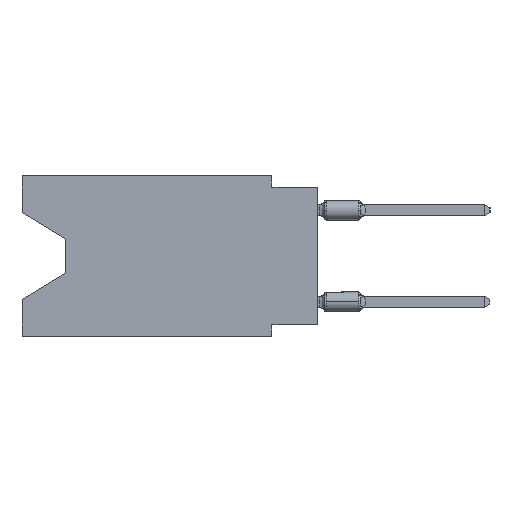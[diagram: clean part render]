
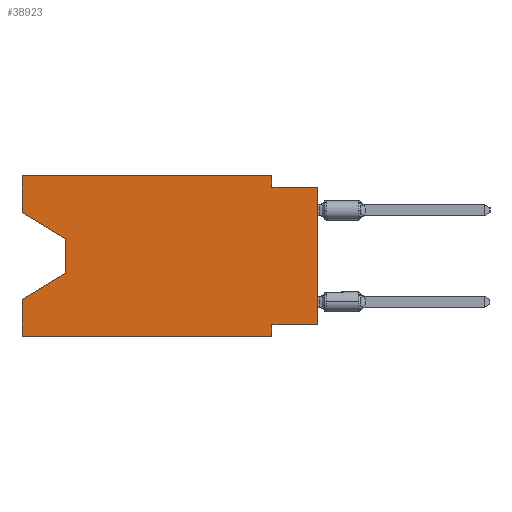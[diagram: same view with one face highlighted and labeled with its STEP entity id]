
A CAD part, left-side view. The second image highlights one B-rep face of the part: STEP entity #38923.
In plain terms, the highlighted planar face has unit normal (-1, 0, 0).
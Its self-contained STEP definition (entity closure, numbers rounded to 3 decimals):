
#684 = EDGE_CURVE ( 'NONE', #58308, #8940, #3826, .T. ) ;
#695 = CARTESIAN_POINT ( 'NONE',  ( 0., 2.54, -8.89 ) ) ;
#1593 = DIRECTION ( 'NONE',  ( 0., -0.855, -0.519 ) ) ;
#2212 = CARTESIAN_POINT ( 'NONE',  ( 0., 16.383, 0. ) ) ;
#3534 = CARTESIAN_POINT ( 'NONE',  ( 0., 0., -8.255 ) ) ;
#3826 = LINE ( 'NONE', #34626, #11736 ) ;
#4796 = CARTESIAN_POINT ( 'NONE',  ( 0., 0., 0. ) ) ;
#4822 = LINE ( 'NONE', #24619, #62692 ) ;
#5678 = ORIENTED_EDGE ( 'NONE', *, *, #39898, .F. ) ;
#6106 = LINE ( 'NONE', #2212, #19301 ) ;
#6407 = CARTESIAN_POINT ( 'NONE',  ( 0., 2.54, 0. ) ) ;
#6414 = ORIENTED_EDGE ( 'NONE', *, *, #52025, .T. ) ;
#8940 = VERTEX_POINT ( 'NONE', #32730 ) ;
#10403 = CARTESIAN_POINT ( 'NONE',  ( 0., 16.383, 0. ) ) ;
#10433 = VECTOR ( 'NONE', #1593, 1000. ) ;
#10930 = ORIENTED_EDGE ( 'NONE', *, *, #32359, .F. ) ;
#10970 = CARTESIAN_POINT ( 'NONE',  ( 0., 2.54, -8.89 ) ) ;
#11038 = VERTEX_POINT ( 'NONE', #6407 ) ;
#11736 = VECTOR ( 'NONE', #29138, 1000. ) ;
#12804 = EDGE_CURVE ( 'NONE', #33223, #33283, #43847, .T. ) ;
#13610 = ORIENTED_EDGE ( 'NONE', *, *, #12804, .F. ) ;
#13977 = DIRECTION ( 'NONE',  ( 0., 0., 1. ) ) ;
#14227 = DIRECTION ( 'NONE',  ( 0., 1., 0. ) ) ;
#14427 = VECTOR ( 'NONE', #24593, 1000. ) ;
#15808 = CARTESIAN_POINT ( 'NONE',  ( 0., 16.383, -8.89 ) ) ;
#15927 = ORIENTED_EDGE ( 'NONE', *, *, #684, .F. ) ;
#17011 = VERTEX_POINT ( 'NONE', #32107 ) ;
#19301 = VECTOR ( 'NONE', #35634, 1000. ) ;
#19447 = DIRECTION ( 'NONE',  ( 0., 0., -1. ) ) ;
#20190 = DIRECTION ( 'NONE',  ( 0., 0., -1. ) ) ;
#22064 = CARTESIAN_POINT ( 'NONE',  ( 0., 16.383, -8.89 ) ) ;
#22142 = VECTOR ( 'NONE', #13977, 1000. ) ;
#22387 = LINE ( 'NONE', #22064, #50321 ) ;
#22866 = CARTESIAN_POINT ( 'NONE',  ( 0., 13.97, -3.505 ) ) ;
#22922 = LINE ( 'NONE', #44001, #56882 ) ;
#24593 = DIRECTION ( 'NONE',  ( 0., 0., 1. ) ) ;
#24619 = CARTESIAN_POINT ( 'NONE',  ( 0., 13.97, -3.505 ) ) ;
#25918 = ORIENTED_EDGE ( 'NONE', *, *, #33167, .T. ) ;
#26257 = LINE ( 'NONE', #51585, #10433 ) ;
#26729 = LINE ( 'NONE', #61464, #43470 ) ;
#27843 = ORIENTED_EDGE ( 'NONE', *, *, #29813, .T. ) ;
#27900 = DIRECTION ( 'NONE',  ( 0., -1., 0. ) ) ;
#27977 = VERTEX_POINT ( 'NONE', #57633 ) ;
#29138 = DIRECTION ( 'NONE',  ( 0., 0., 1. ) ) ;
#29785 = LINE ( 'NONE', #4796, #14427 ) ;
#29813 = EDGE_CURVE ( 'NONE', #63937, #17011, #29785, .T. ) ;
#30918 = VERTEX_POINT ( 'NONE', #59680 ) ;
#32107 = CARTESIAN_POINT ( 'NONE',  ( 0., 0., -0.635 ) ) ;
#32359 = EDGE_CURVE ( 'NONE', #11038, #30918, #26729, .T. ) ;
#32730 = CARTESIAN_POINT ( 'NONE',  ( 0., 16.383, -6.852 ) ) ;
#33167 = EDGE_CURVE ( 'NONE', #33223, #48048, #26257, .T. ) ;
#33223 = VERTEX_POINT ( 'NONE', #33697 ) ;
#33283 = VERTEX_POINT ( 'NONE', #57730 ) ;
#33572 = VECTOR ( 'NONE', #54326, 1000. ) ;
#33697 = CARTESIAN_POINT ( 'NONE',  ( 0., 16.383, -2.038 ) ) ;
#34626 = CARTESIAN_POINT ( 'NONE',  ( 0., 16.383, 0. ) ) ;
#35634 = DIRECTION ( 'NONE',  ( 0., -1., 0. ) ) ;
#36763 = DIRECTION ( 'NONE',  ( 0., 0., -1. ) ) ;
#37464 = ORIENTED_EDGE ( 'NONE', *, *, #62805, .F. ) ;
#38060 = PLANE ( 'NONE',  #52364 ) ;
#38923 = ADVANCED_FACE ( 'NONE', ( #61458 ), #38060, .F. ) ;
#39385 = LINE ( 'NONE', #53347, #33572 ) ;
#39884 = VERTEX_POINT ( 'NONE', #10970 ) ;
#39898 = EDGE_CURVE ( 'NONE', #33283, #11038, #6106, .T. ) ;
#42296 = DIRECTION ( 'NONE',  ( 0., 0., -1. ) ) ;
#42402 = EDGE_CURVE ( 'NONE', #27977, #39884, #59467, .T. ) ;
#43470 = VECTOR ( 'NONE', #42296, 1000. ) ;
#43847 = LINE ( 'NONE', #10403, #22142 ) ;
#44001 = CARTESIAN_POINT ( 'NONE',  ( 0., 0., -0.635 ) ) ;
#46879 = CARTESIAN_POINT ( 'NONE',  ( 0., 13.97, -5.385 ) ) ;
#48005 = LINE ( 'NONE', #3534, #57477 ) ;
#48048 = VERTEX_POINT ( 'NONE', #22866 ) ;
#48259 = ORIENTED_EDGE ( 'NONE', *, *, #62877, .T. ) ;
#50321 = VECTOR ( 'NONE', #27900, 1000. ) ;
#51585 = CARTESIAN_POINT ( 'NONE',  ( 0., 16.383, -2.038 ) ) ;
#52025 = EDGE_CURVE ( 'NONE', #58308, #39884, #22387, .T. ) ;
#52364 = AXIS2_PLACEMENT_3D ( 'NONE', #56901, #61787, #36763 ) ;
#52650 = EDGE_LOOP ( 'NONE', ( #25918, #48259, #57878, #15927, #6414, #63016, #37464, #27843, #53165, #10930, #5678, #13610 ) ) ;
#53165 = ORIENTED_EDGE ( 'NONE', *, *, #57489, .F. ) ;
#53347 = CARTESIAN_POINT ( 'NONE',  ( 0., 13.97, -5.385 ) ) ;
#54091 = DIRECTION ( 'NONE',  ( 0., -1., 0. ) ) ;
#54326 = DIRECTION ( 'NONE',  ( 0., 0.855, -0.519 ) ) ;
#55642 = VERTEX_POINT ( 'NONE', #46879 ) ;
#56033 = CARTESIAN_POINT ( 'NONE',  ( 0., 0., -8.255 ) ) ;
#56882 = VECTOR ( 'NONE', #54091, 1000. ) ;
#56901 = CARTESIAN_POINT ( 'NONE',  ( 0., 16.383, 0. ) ) ;
#57477 = VECTOR ( 'NONE', #14227, 1000. ) ;
#57489 = EDGE_CURVE ( 'NONE', #30918, #17011, #22922, .T. ) ;
#57633 = CARTESIAN_POINT ( 'NONE',  ( 0., 2.54, -8.255 ) ) ;
#57730 = CARTESIAN_POINT ( 'NONE',  ( 0., 16.383, 0. ) ) ;
#57878 = ORIENTED_EDGE ( 'NONE', *, *, #62018, .T. ) ;
#58308 = VERTEX_POINT ( 'NONE', #15808 ) ;
#59467 = LINE ( 'NONE', #695, #59980 ) ;
#59680 = CARTESIAN_POINT ( 'NONE',  ( 0., 2.54, -0.635 ) ) ;
#59980 = VECTOR ( 'NONE', #20190, 1000. ) ;
#61458 = FACE_OUTER_BOUND ( 'NONE', #52650, .T. ) ;
#61464 = CARTESIAN_POINT ( 'NONE',  ( 0., 2.54, 0. ) ) ;
#61787 = DIRECTION ( 'NONE',  ( 1., 0., 0. ) ) ;
#62018 = EDGE_CURVE ( 'NONE', #55642, #8940, #39385, .T. ) ;
#62692 = VECTOR ( 'NONE', #19447, 1000. ) ;
#62805 = EDGE_CURVE ( 'NONE', #63937, #27977, #48005, .T. ) ;
#62877 = EDGE_CURVE ( 'NONE', #48048, #55642, #4822, .T. ) ;
#63016 = ORIENTED_EDGE ( 'NONE', *, *, #42402, .F. ) ;
#63937 = VERTEX_POINT ( 'NONE', #56033 ) ;
